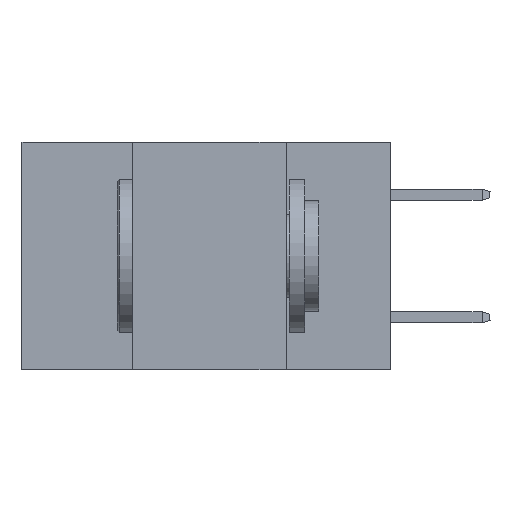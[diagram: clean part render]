
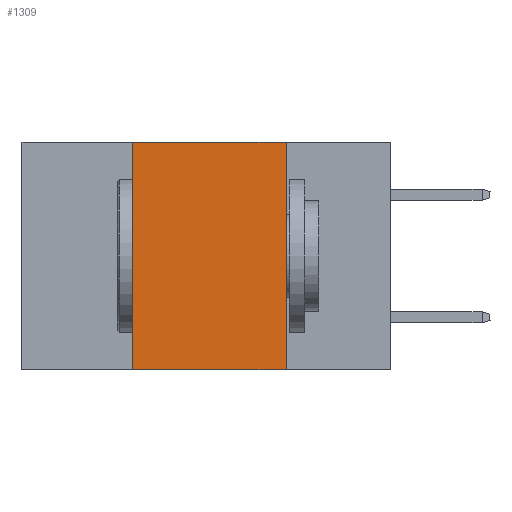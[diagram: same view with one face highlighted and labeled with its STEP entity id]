
A CAD part, left-side view. The second image highlights one B-rep face of the part: STEP entity #1309.
In plain terms, the highlighted planar face has unit normal (-1, 0, 0).
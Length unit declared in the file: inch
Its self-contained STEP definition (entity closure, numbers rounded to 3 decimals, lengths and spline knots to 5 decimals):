
#150 = VERTEX_POINT ( 'NONE', #19500 ) ;
#793 = VECTOR ( 'NONE', #15546, 39.37008 ) ;
#1051 = EDGE_CURVE ( 'NONE', #9261, #150, #17961, .T. ) ;
#1309 = ADVANCED_FACE ( 'NONE', ( #7633 ), #21838, .F. ) ;
#1480 = DIRECTION ( 'NONE',  ( 0., 0., 1. ) ) ;
#3304 = CARTESIAN_POINT ( 'NONE',  ( 0., 0.42, -0.37 ) ) ;
#5239 = ORIENTED_EDGE ( 'NONE', *, *, #13242, .F. ) ;
#6891 = EDGE_LOOP ( 'NONE', ( #18402, #5239, #14766, #15342 ) ) ;
#7633 = FACE_OUTER_BOUND ( 'NONE', #6891, .T. ) ;
#8812 = LINE ( 'NONE', #17705, #17739 ) ;
#8918 = LINE ( 'NONE', #13564, #18416 ) ;
#9001 = EDGE_CURVE ( 'NONE', #10000, #150, #8918, .T. ) ;
#9261 = VERTEX_POINT ( 'NONE', #19368 ) ;
#9995 = DIRECTION ( 'NONE',  ( 0., -1., 0. ) ) ;
#10000 = VERTEX_POINT ( 'NONE', #3304 ) ;
#11300 = EDGE_CURVE ( 'NONE', #10000, #11490, #8812, .T. ) ;
#11490 = VERTEX_POINT ( 'NONE', #20458 ) ;
#11516 = AXIS2_PLACEMENT_3D ( 'NONE', #21807, #21672, #21634 ) ;
#13242 = EDGE_CURVE ( 'NONE', #11490, #9261, #19434, .T. ) ;
#13564 = CARTESIAN_POINT ( 'NONE',  ( 0., 0.6, -0.37 ) ) ;
#14766 = ORIENTED_EDGE ( 'NONE', *, *, #11300, .F. ) ;
#15342 = ORIENTED_EDGE ( 'NONE', *, *, #9001, .T. ) ;
#15546 = DIRECTION ( 'NONE',  ( 0., -1., 0. ) ) ;
#17705 = CARTESIAN_POINT ( 'NONE',  ( 0., 0.42, 0. ) ) ;
#17718 = DIRECTION ( 'NONE',  ( 0., 0., -1. ) ) ;
#17739 = VECTOR ( 'NONE', #1480, 39.37008 ) ;
#17791 = CARTESIAN_POINT ( 'NONE',  ( 0., 0.17, 0. ) ) ;
#17961 = LINE ( 'NONE', #17791, #22750 ) ;
#18402 = ORIENTED_EDGE ( 'NONE', *, *, #1051, .F. ) ;
#18416 = VECTOR ( 'NONE', #9995, 39.37008 ) ;
#19055 = CARTESIAN_POINT ( 'NONE',  ( 0., 0.6, 0. ) ) ;
#19368 = CARTESIAN_POINT ( 'NONE',  ( 0., 0.17, 0. ) ) ;
#19434 = LINE ( 'NONE', #19055, #793 ) ;
#19500 = CARTESIAN_POINT ( 'NONE',  ( 0., 0.17, -0.37 ) ) ;
#20458 = CARTESIAN_POINT ( 'NONE',  ( 0., 0.42, 0. ) ) ;
#21634 = DIRECTION ( 'NONE',  ( 0., 0., -1. ) ) ;
#21672 = DIRECTION ( 'NONE',  ( 1., 0., 0. ) ) ;
#21807 = CARTESIAN_POINT ( 'NONE',  ( 0., 0.6, 0. ) ) ;
#21838 = PLANE ( 'NONE',  #11516 ) ;
#22750 = VECTOR ( 'NONE', #17718, 39.37008 ) ;
